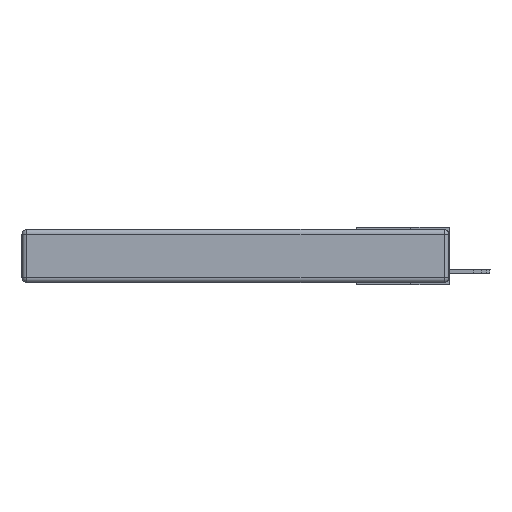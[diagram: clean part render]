
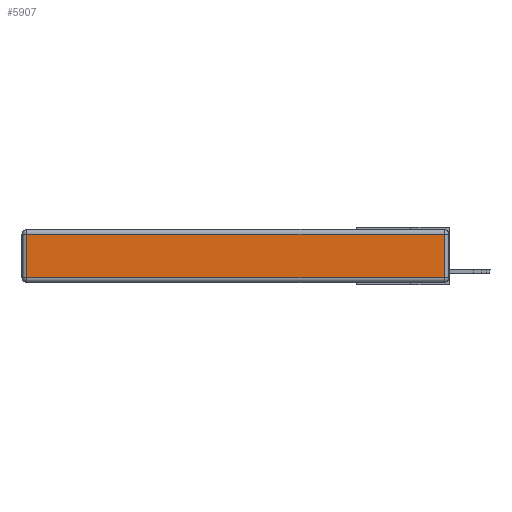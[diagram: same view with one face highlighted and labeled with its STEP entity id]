
A CAD part, left-side view. The second image highlights one B-rep face of the part: STEP entity #5907.
In plain terms, the highlighted planar face has unit normal (-1, 0, 0).
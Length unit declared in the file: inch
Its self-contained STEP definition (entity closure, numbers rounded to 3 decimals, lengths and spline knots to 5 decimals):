
#508 = VERTEX_POINT ( 'NONE', #13134 ) ;
#875 = VERTEX_POINT ( 'NONE', #5504 ) ;
#1112 = LINE ( 'NONE', #7741, #11164 ) ;
#1545 = FACE_OUTER_BOUND ( 'NONE', #4578, .T. ) ;
#2048 = ORIENTED_EDGE ( 'NONE', *, *, #14444, .T. ) ;
#2552 = DIRECTION ( 'NONE',  ( 0., 0., 1. ) ) ;
#2832 = VECTOR ( 'NONE', #12604, 39.37008 ) ;
#4578 = EDGE_LOOP ( 'NONE', ( #2048, #9298, #5114, #7653 ) ) ;
#4933 = EDGE_CURVE ( 'NONE', #875, #9102, #14356, .T. ) ;
#5114 = ORIENTED_EDGE ( 'NONE', *, *, #6490, .T. ) ;
#5504 = CARTESIAN_POINT ( 'NONE',  ( 0., 2.72, -0.03 ) ) ;
#5589 = AXIS2_PLACEMENT_3D ( 'NONE', #14320, #7842, #2552 ) ;
#5907 = ADVANCED_FACE ( 'NONE', ( #1545 ), #10589, .T. ) ;
#6233 = DIRECTION ( 'NONE',  ( 0., 1., 0. ) ) ;
#6490 = EDGE_CURVE ( 'NONE', #508, #875, #1112, .T. ) ;
#7043 = LINE ( 'NONE', #8377, #16028 ) ;
#7099 = VERTEX_POINT ( 'NONE', #14591 ) ;
#7208 = DIRECTION ( 'NONE',  ( 0., -1., 0. ) ) ;
#7653 = ORIENTED_EDGE ( 'NONE', *, *, #4933, .T. ) ;
#7741 = CARTESIAN_POINT ( 'NONE',  ( 0., 2.75, -0.03 ) ) ;
#7842 = DIRECTION ( 'NONE',  ( -1., 0., 0. ) ) ;
#8377 = CARTESIAN_POINT ( 'NONE',  ( 0., 0., -0.313 ) ) ;
#8622 = CARTESIAN_POINT ( 'NONE',  ( 0., 2.72, -0.343 ) ) ;
#8881 = LINE ( 'NONE', #12244, #15590 ) ;
#9102 = VERTEX_POINT ( 'NONE', #15632 ) ;
#9298 = ORIENTED_EDGE ( 'NONE', *, *, #15276, .T. ) ;
#10589 = PLANE ( 'NONE',  #5589 ) ;
#11164 = VECTOR ( 'NONE', #6233, 39.37008 ) ;
#12244 = CARTESIAN_POINT ( 'NONE',  ( 0., 0.03, -0.343 ) ) ;
#12604 = DIRECTION ( 'NONE',  ( 0., 0., -1. ) ) ;
#13134 = CARTESIAN_POINT ( 'NONE',  ( 0., 0.03, -0.03 ) ) ;
#13647 = DIRECTION ( 'NONE',  ( 0., 0., 1. ) ) ;
#14320 = CARTESIAN_POINT ( 'NONE',  ( 0., 0., -0.343 ) ) ;
#14356 = LINE ( 'NONE', #8622, #2832 ) ;
#14444 = EDGE_CURVE ( 'NONE', #9102, #7099, #7043, .T. ) ;
#14591 = CARTESIAN_POINT ( 'NONE',  ( 0., 0.03, -0.313 ) ) ;
#15276 = EDGE_CURVE ( 'NONE', #7099, #508, #8881, .T. ) ;
#15590 = VECTOR ( 'NONE', #13647, 39.37008 ) ;
#15632 = CARTESIAN_POINT ( 'NONE',  ( 0., 2.72, -0.313 ) ) ;
#16028 = VECTOR ( 'NONE', #7208, 39.37008 ) ;
